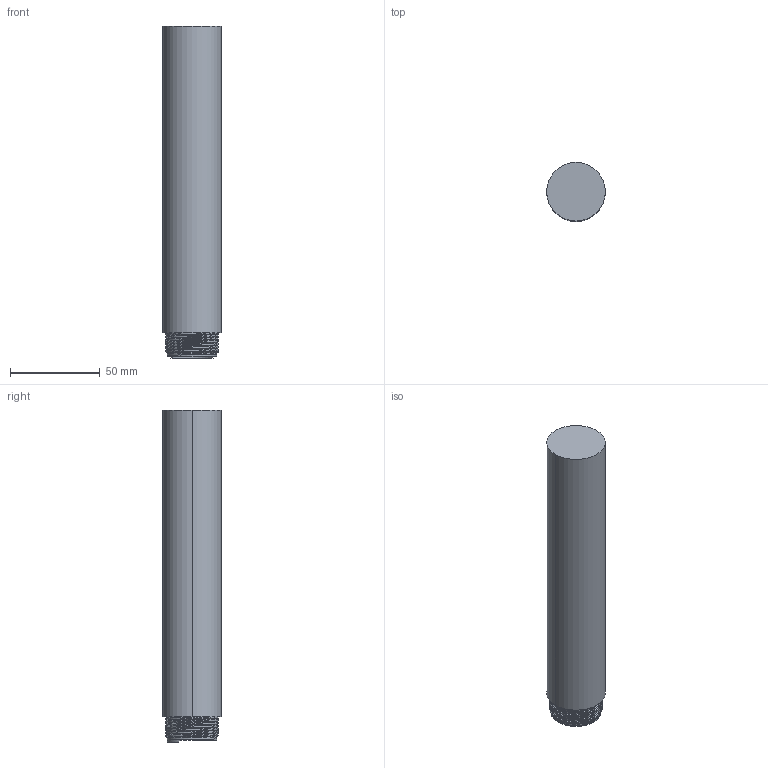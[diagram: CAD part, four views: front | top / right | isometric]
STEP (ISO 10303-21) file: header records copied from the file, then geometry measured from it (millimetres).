
FILE_DESCRIPTION (( 'STEP AP214' ), '1' );
FILE_NAME ('P-15_Tube.STEP', '2013-12-11T21:34:13', ( 'elpi' ), ( '' ), 'SwSTEP 2.0', 'SolidWorks 2013', '' );
FILE_SCHEMA (( 'AUTOMOTIVE_DESIGN' ));
Length unit declared in the file: inch
Products named in the file (1): P-15_Tube
Bounding box: 32.77 x 32.77 x 185.42 mm (x, y, z)
Volume: 62856.5 mm3; surface area: 35267.1 mm2
Topology: 1 solids, 1 shells, 84 faces, 243 edges, 162 vertices
Faces by surface type: cylinder 39, plane 23, bspline 18, cone 4
Entity records: 8089 total; most frequent: CARTESIAN_POINT 6281, ORIENTED_EDGE 486, EDGE_CURVE 243, DIRECTION 243, VERTEX_POINT 162, AXIS2_PLACEMENT_3D 91, EDGE_LOOP 85, FACE_OUTER_BOUND 84
